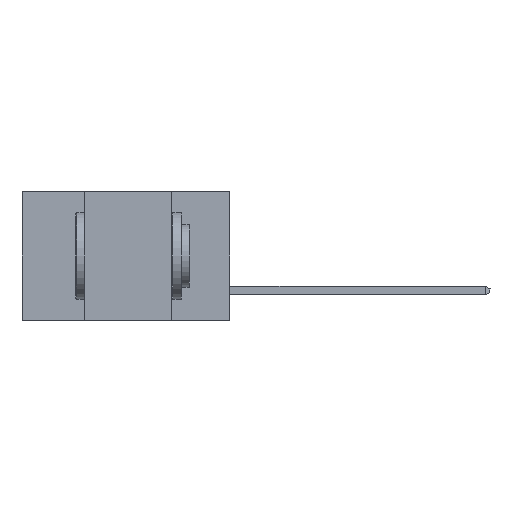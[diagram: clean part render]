
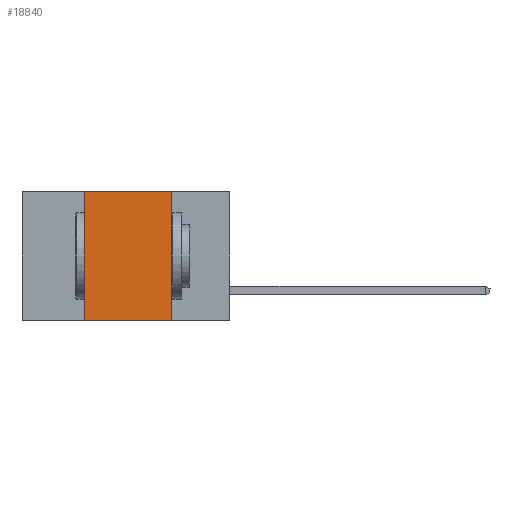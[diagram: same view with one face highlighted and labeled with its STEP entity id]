
A CAD part, left-side view. The second image highlights one B-rep face of the part: STEP entity #18840.
In plain terms, the highlighted planar face has unit normal (-1, 0, 0).
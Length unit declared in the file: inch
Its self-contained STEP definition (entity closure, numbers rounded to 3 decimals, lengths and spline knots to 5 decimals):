
#1916 = PLANE ( 'NONE',  #6649 ) ;
#2316 = CARTESIAN_POINT ( 'NONE',  ( 0., 0.17, -0.37 ) ) ;
#2713 = CARTESIAN_POINT ( 'NONE',  ( 0., 0.17, 0. ) ) ;
#3500 = VECTOR ( 'NONE', #9757, 39.37008 ) ;
#3868 = LINE ( 'NONE', #5619, #12637 ) ;
#5335 = ORIENTED_EDGE ( 'NONE', *, *, #7515, .F. ) ;
#5417 = EDGE_CURVE ( 'NONE', #19298, #9909, #15733, .T. ) ;
#5500 = CARTESIAN_POINT ( 'NONE',  ( 0., 0.42, 0. ) ) ;
#5515 = CARTESIAN_POINT ( 'NONE',  ( 0., 0.42, -0.37 ) ) ;
#5619 = CARTESIAN_POINT ( 'NONE',  ( 0., 0.6, -0.37 ) ) ;
#6505 = LINE ( 'NONE', #13025, #14701 ) ;
#6614 = CARTESIAN_POINT ( 'NONE',  ( 0., 0.6, 0. ) ) ;
#6649 = AXIS2_PLACEMENT_3D ( 'NONE', #15286, #20071, #20192 ) ;
#6768 = ORIENTED_EDGE ( 'NONE', *, *, #12850, .T. ) ;
#7515 = EDGE_CURVE ( 'NONE', #9909, #11773, #7929, .T. ) ;
#7532 = EDGE_LOOP ( 'NONE', ( #16743, #5335, #11300, #6768 ) ) ;
#7929 = LINE ( 'NONE', #6614, #3500 ) ;
#9622 = DIRECTION ( 'NONE',  ( 0., 0., -1. ) ) ;
#9757 = DIRECTION ( 'NONE',  ( 0., -1., 0. ) ) ;
#9909 = VERTEX_POINT ( 'NONE', #5500 ) ;
#11300 = ORIENTED_EDGE ( 'NONE', *, *, #5417, .F. ) ;
#11773 = VERTEX_POINT ( 'NONE', #2713 ) ;
#12235 = DIRECTION ( 'NONE',  ( 0., -1., 0. ) ) ;
#12637 = VECTOR ( 'NONE', #12235, 39.37008 ) ;
#12850 = EDGE_CURVE ( 'NONE', #19298, #19351, #3868, .T. ) ;
#13025 = CARTESIAN_POINT ( 'NONE',  ( 0., 0.17, -0.37 ) ) ;
#13441 = FACE_OUTER_BOUND ( 'NONE', #7532, .T. ) ;
#14162 = CARTESIAN_POINT ( 'NONE',  ( 0., 0.42, -0.37 ) ) ;
#14701 = VECTOR ( 'NONE', #9622, 39.37008 ) ;
#15286 = CARTESIAN_POINT ( 'NONE',  ( 0., 0.6, 0. ) ) ;
#15733 = LINE ( 'NONE', #5515, #17710 ) ;
#15771 = EDGE_CURVE ( 'NONE', #11773, #19351, #6505, .T. ) ;
#16743 = ORIENTED_EDGE ( 'NONE', *, *, #15771, .F. ) ;
#17710 = VECTOR ( 'NONE', #20511, 39.37008 ) ;
#18840 = ADVANCED_FACE ( 'NONE', ( #13441 ), #1916, .F. ) ;
#19298 = VERTEX_POINT ( 'NONE', #14162 ) ;
#19351 = VERTEX_POINT ( 'NONE', #2316 ) ;
#20071 = DIRECTION ( 'NONE',  ( 1., 0., 0. ) ) ;
#20192 = DIRECTION ( 'NONE',  ( 0., 0., -1. ) ) ;
#20511 = DIRECTION ( 'NONE',  ( 0., 0., 1. ) ) ;
